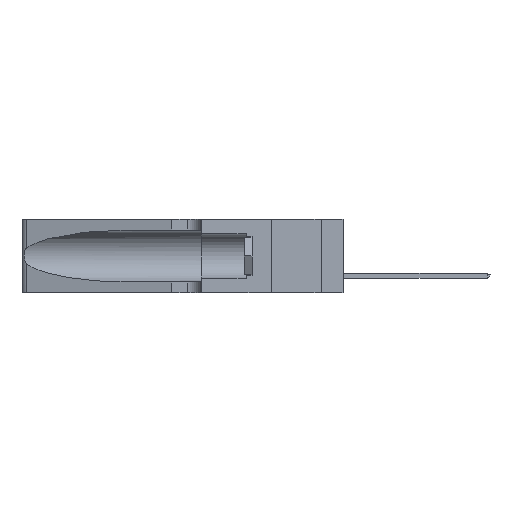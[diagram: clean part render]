
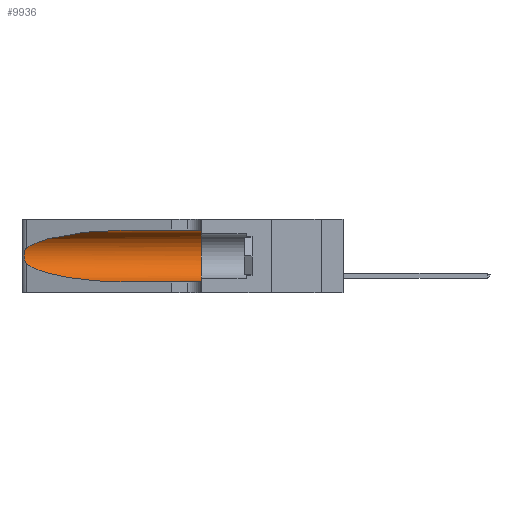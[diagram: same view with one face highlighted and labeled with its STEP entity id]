
A CAD part, left-side view. The second image highlights one B-rep face of the part: STEP entity #9936.
In plain terms, the highlighted cylindrical face has radius 3.308 mm (diameter 6.617 mm), a partial arc.
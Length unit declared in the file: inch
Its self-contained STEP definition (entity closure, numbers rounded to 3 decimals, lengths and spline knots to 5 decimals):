
#912 = CARTESIAN_POINT ( 'NONE',  ( 0.25487, 1.22718, 0.14631 ) ) ;
#1186 = ORIENTED_EDGE ( 'NONE', *, *, #17201, .F. ) ;
#2147 = LINE ( 'NONE', #11104, #3465 ) ;
#2642 = ORIENTED_EDGE ( 'NONE', *, *, #5126, .T. ) ;
#3251 =( BOUNDED_CURVE ( )  B_SPLINE_CURVE ( 3, ( #912, #8893, #5035, #30622 ),
 .UNSPECIFIED., .F., .F. ) 
 B_SPLINE_CURVE_WITH_KNOTS ( ( 4, 4 ),
 ( 3.44316, 4.71239 ),
 .UNSPECIFIED. ) 
 CURVE ( )  GEOMETRIC_REPRESENTATION_ITEM ( )  RATIONAL_B_SPLINE_CURVE ( ( 1., 0.87, 0.87, 1. ) ) 
 REPRESENTATION_ITEM ( '' )  );
#3465 = VECTOR ( 'NONE', #31210, 39.37008 ) ;
#4172 = VERTEX_POINT ( 'NONE', #6641 ) ;
#5035 = CARTESIAN_POINT ( 'NONE',  ( 0.18966, 0.96281, 0.05475 ) ) ;
#5126 = EDGE_CURVE ( 'NONE', #4172, #24349, #2147, .T. ) ;
#5612 = DIRECTION ( 'NONE',  ( 0., 0., -1. ) ) ;
#6641 = CARTESIAN_POINT ( 'NONE',  ( 0.1305, 0.72297, 0.05475 ) ) ;
#7658 = DIRECTION ( 'NONE',  ( 0., 0., 1. ) ) ;
#8053 = VERTEX_POINT ( 'NONE', #41921 ) ;
#8138 = CARTESIAN_POINT ( 'NONE',  ( 0.1305, 1.61858, 0.31525 ) ) ;
#8893 = CARTESIAN_POINT ( 'NONE',  ( 0.2373, 1.15595, 0.08982 ) ) ;
#9936 = ADVANCED_FACE ( 'NONE', ( #11574 ), #19623, .F. ) ;
#10081 = VERTEX_POINT ( 'NONE', #19114 ) ;
#10957 = CARTESIAN_POINT ( 'NONE',  ( 0.25789, 1.23486, 0.15765 ) ) ;
#11104 = CARTESIAN_POINT ( 'NONE',  ( 0.1305, 1.61858, 0.05475 ) ) ;
#11574 = FACE_OUTER_BOUND ( 'NONE', #43544, .T. ) ;
#12359 = CARTESIAN_POINT ( 'NONE',  ( 0.25487, 1.22718, 0.22369 ) ) ;
#12375 = B_SPLINE_CURVE_WITH_KNOTS ( 'NONE', 3,
 ( #26868, #42667, #41953, #26133, #30529, #38323, #30895, #14605, #14788, #18170, #10957, #34884, #42310, #18928 ),
 .UNSPECIFIED., .F., .F.,
 ( 4, 2, 2, 2, 2, 2, 4 ),
 ( 0., 0.00027, 0.00053, 0.00107, 0.0016, 0.00187, 0.00214 ),
 .UNSPECIFIED. ) ;
#12769 = CARTESIAN_POINT ( 'NONE',  ( 0.1305, 1.61858, 0.185 ) ) ;
#14605 = CARTESIAN_POINT ( 'NONE',  ( 0.26075, 1.23896, 0.178 ) ) ;
#14788 = CARTESIAN_POINT ( 'NONE',  ( 0.26017, 1.23833, 0.17102 ) ) ;
#16990 = CIRCLE ( 'NONE', #46869, 0.13025 ) ;
#17201 = EDGE_CURVE ( 'NONE', #8053, #24349, #16990, .T. ) ;
#18170 = CARTESIAN_POINT ( 'NONE',  ( 0.25856, 1.23593, 0.16098 ) ) ;
#18334 = VECTOR ( 'NONE', #43815, 39.37008 ) ;
#18928 = CARTESIAN_POINT ( 'NONE',  ( 0.25487, 1.22718, 0.14631 ) ) ;
#19114 = CARTESIAN_POINT ( 'NONE',  ( 0.1305, 0.72297, 0.31525 ) ) ;
#19274 = CARTESIAN_POINT ( 'NONE',  ( 0.1305, 0.35, 0.185 ) ) ;
#19623 = CYLINDRICAL_SURFACE ( 'NONE', #43697, 0.13025 ) ;
#20042 = ORIENTED_EDGE ( 'NONE', *, *, #28234, .F. ) ;
#21223 = EDGE_CURVE ( 'NONE', #10081, #30991, #32342, .T. ) ;
#22898 = ORIENTED_EDGE ( 'NONE', *, *, #29448, .T. ) ;
#24014 = CARTESIAN_POINT ( 'NONE',  ( 0.1305, 0.35, 0.05475 ) ) ;
#24349 = VERTEX_POINT ( 'NONE', #24014 ) ;
#26133 = CARTESIAN_POINT ( 'NONE',  ( 0.25787, 1.23484, 0.2124 ) ) ;
#26868 = CARTESIAN_POINT ( 'NONE',  ( 0.25487, 1.22718, 0.22369 ) ) ;
#28103 = VERTEX_POINT ( 'NONE', #41870 ) ;
#28234 = EDGE_CURVE ( 'NONE', #10081, #8053, #38180, .T. ) ;
#29448 = EDGE_CURVE ( 'NONE', #30991, #28103, #12375, .T. ) ;
#29624 = CARTESIAN_POINT ( 'NONE',  ( 0.2373, 1.15595, 0.28018 ) ) ;
#30529 = CARTESIAN_POINT ( 'NONE',  ( 0.25854, 1.2359, 0.20912 ) ) ;
#30622 = CARTESIAN_POINT ( 'NONE',  ( 0.1305, 0.72297, 0.05475 ) ) ;
#30895 = CARTESIAN_POINT ( 'NONE',  ( 0.26075, 1.23896, 0.19203 ) ) ;
#30991 = VERTEX_POINT ( 'NONE', #12359 ) ;
#31210 = DIRECTION ( 'NONE',  ( 0., -1., 0. ) ) ;
#31412 = DIRECTION ( 'NONE',  ( 0., 1., 0. ) ) ;
#31424 = ORIENTED_EDGE ( 'NONE', *, *, #21223, .T. ) ;
#32342 =( BOUNDED_CURVE ( )  B_SPLINE_CURVE ( 3, ( #34392, #42359, #29624, #33634 ),
 .UNSPECIFIED., .F., .F. ) 
 B_SPLINE_CURVE_WITH_KNOTS ( ( 4, 4 ),
 ( 1.5708, 2.84003 ),
 .UNSPECIFIED. ) 
 CURVE ( )  GEOMETRIC_REPRESENTATION_ITEM ( )  RATIONAL_B_SPLINE_CURVE ( ( 1., 0.87, 0.87, 1. ) ) 
 REPRESENTATION_ITEM ( '' )  );
#33272 = EDGE_CURVE ( 'NONE', #28103, #4172, #3251, .T. ) ;
#33634 = CARTESIAN_POINT ( 'NONE',  ( 0.25487, 1.22718, 0.22369 ) ) ;
#34392 = CARTESIAN_POINT ( 'NONE',  ( 0.1305, 0.72297, 0.31525 ) ) ;
#34884 = CARTESIAN_POINT ( 'NONE',  ( 0.25639, 1.23186, 0.15144 ) ) ;
#37168 = DIRECTION ( 'NONE',  ( 0., -1., 0. ) ) ;
#38180 = LINE ( 'NONE', #8138, #18334 ) ;
#38323 = CARTESIAN_POINT ( 'NONE',  ( 0.26018, 1.23835, 0.19895 ) ) ;
#41870 = CARTESIAN_POINT ( 'NONE',  ( 0.25487, 1.22718, 0.14631 ) ) ;
#41921 = CARTESIAN_POINT ( 'NONE',  ( 0.1305, 0.35, 0.31525 ) ) ;
#41953 = CARTESIAN_POINT ( 'NONE',  ( 0.25639, 1.23184, 0.21858 ) ) ;
#42310 = CARTESIAN_POINT ( 'NONE',  ( 0.25555, 1.22993, 0.14849 ) ) ;
#42359 = CARTESIAN_POINT ( 'NONE',  ( 0.18966, 0.96281, 0.31525 ) ) ;
#42667 = CARTESIAN_POINT ( 'NONE',  ( 0.25555, 1.22994, 0.2215 ) ) ;
#43276 = ORIENTED_EDGE ( 'NONE', *, *, #33272, .T. ) ;
#43544 = EDGE_LOOP ( 'NONE', ( #31424, #22898, #43276, #2642, #1186, #20042 ) ) ;
#43697 = AXIS2_PLACEMENT_3D ( 'NONE', #12769, #37168, #5612 ) ;
#43815 = DIRECTION ( 'NONE',  ( 0., -1., 0. ) ) ;
#46869 = AXIS2_PLACEMENT_3D ( 'NONE', #19274, #31412, #7658 ) ;
